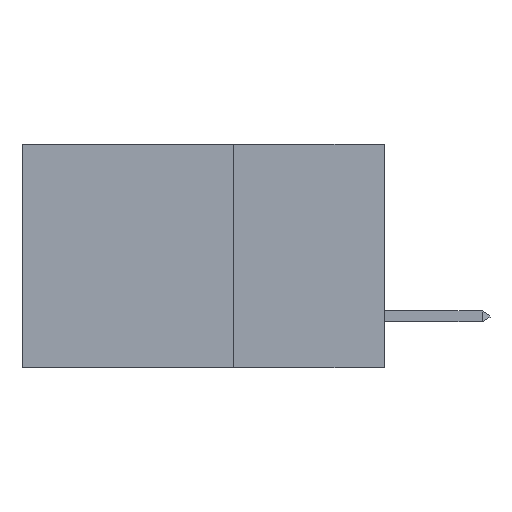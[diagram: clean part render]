
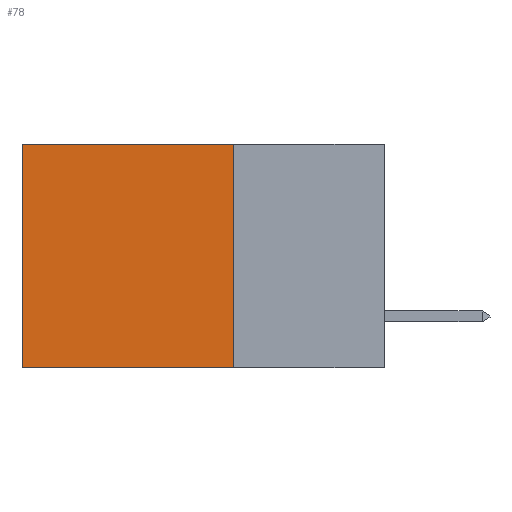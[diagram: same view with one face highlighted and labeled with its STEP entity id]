
A CAD part, left-side view. The second image highlights one B-rep face of the part: STEP entity #78.
In plain terms, the highlighted planar face has unit normal (-1, 0, 0).
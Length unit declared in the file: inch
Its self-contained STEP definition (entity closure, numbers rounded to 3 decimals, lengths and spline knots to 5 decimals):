
#78 = ADVANCED_FACE ( 'NONE', ( #19194 ), #13484, .F. ) ;
#245 = EDGE_CURVE ( 'NONE', #12605, #11792, #19489, .T. ) ;
#565 = LINE ( 'NONE', #12277, #20907 ) ;
#1634 = CARTESIAN_POINT ( 'NONE',  ( 0.2875, 0.6, 0. ) ) ;
#1679 = VECTOR ( 'NONE', #10312, 39.37008 ) ;
#2183 = ORIENTED_EDGE ( 'NONE', *, *, #21502, .T. ) ;
#3192 = CARTESIAN_POINT ( 'NONE',  ( 0.2875, 0.6, -0.37 ) ) ;
#3549 = ORIENTED_EDGE ( 'NONE', *, *, #12473, .F. ) ;
#4205 = EDGE_CURVE ( 'NONE', #12605, #25446, #22047, .T. ) ;
#4560 = DIRECTION ( 'NONE',  ( 0., 0., -1. ) ) ;
#4764 = VERTEX_POINT ( 'NONE', #3192 ) ;
#7401 = AXIS2_PLACEMENT_3D ( 'NONE', #19480, #20046, #9251 ) ;
#9251 = DIRECTION ( 'NONE',  ( 0., 0., -1. ) ) ;
#10312 = DIRECTION ( 'NONE',  ( 0., 1., 0. ) ) ;
#11011 = CARTESIAN_POINT ( 'NONE',  ( 0.2875, 0.25, 0. ) ) ;
#11629 = VECTOR ( 'NONE', #17305, 39.37008 ) ;
#11792 = VERTEX_POINT ( 'NONE', #16161 ) ;
#12277 = CARTESIAN_POINT ( 'NONE',  ( 0.2875, 0.6, 0. ) ) ;
#12473 = EDGE_CURVE ( 'NONE', #11792, #4764, #23249, .T. ) ;
#12605 = VERTEX_POINT ( 'NONE', #18557 ) ;
#13484 = PLANE ( 'NONE',  #7401 ) ;
#13789 = ORIENTED_EDGE ( 'NONE', *, *, #245, .F. ) ;
#14615 = CARTESIAN_POINT ( 'NONE',  ( 0.2875, 0.25, 0. ) ) ;
#16161 = CARTESIAN_POINT ( 'NONE',  ( 0.2875, 0.25, -0.37 ) ) ;
#16846 = ORIENTED_EDGE ( 'NONE', *, *, #4205, .T. ) ;
#17010 = EDGE_LOOP ( 'NONE', ( #2183, #3549, #13789, #16846 ) ) ;
#17305 = DIRECTION ( 'NONE',  ( 0., 1., 0. ) ) ;
#18557 = CARTESIAN_POINT ( 'NONE',  ( 0.2875, 0.25, 0. ) ) ;
#19194 = FACE_OUTER_BOUND ( 'NONE', #17010, .T. ) ;
#19480 = CARTESIAN_POINT ( 'NONE',  ( 0.2875, 0.25, 0. ) ) ;
#19489 = LINE ( 'NONE', #14615, #25318 ) ;
#20046 = DIRECTION ( 'NONE',  ( 1., 0., 0. ) ) ;
#20100 = CARTESIAN_POINT ( 'NONE',  ( 0.2875, 0.25, -0.37 ) ) ;
#20152 = DIRECTION ( 'NONE',  ( 0., 0., -1. ) ) ;
#20907 = VECTOR ( 'NONE', #20152, 39.37008 ) ;
#21502 = EDGE_CURVE ( 'NONE', #25446, #4764, #565, .T. ) ;
#22047 = LINE ( 'NONE', #11011, #11629 ) ;
#23249 = LINE ( 'NONE', #20100, #1679 ) ;
#25318 = VECTOR ( 'NONE', #4560, 39.37008 ) ;
#25446 = VERTEX_POINT ( 'NONE', #1634 ) ;
